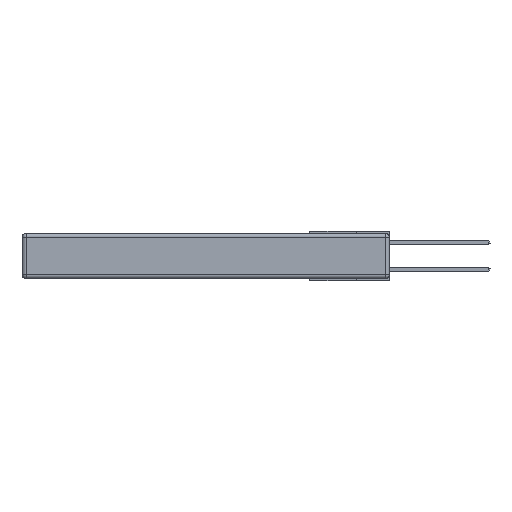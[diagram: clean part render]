
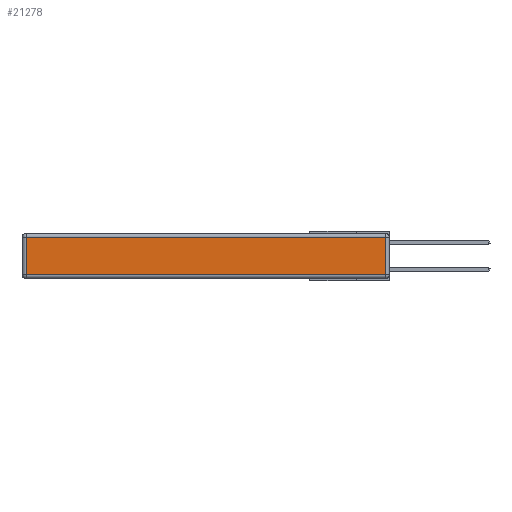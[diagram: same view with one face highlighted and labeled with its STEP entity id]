
A CAD part, left-side view. The second image highlights one B-rep face of the part: STEP entity #21278.
In plain terms, the highlighted planar face has unit normal (-1, 0, 0).
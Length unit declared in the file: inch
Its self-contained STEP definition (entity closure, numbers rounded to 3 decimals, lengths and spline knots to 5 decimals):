
#412 = ORIENTED_EDGE ( 'NONE', *, *, #29593, .T. ) ;
#1567 = VECTOR ( 'NONE', #12972, 39.37008 ) ;
#4146 = DIRECTION ( 'NONE',  ( -1., 0., 0. ) ) ;
#5106 = ORIENTED_EDGE ( 'NONE', *, *, #32100, .T. ) ;
#6417 = EDGE_LOOP ( 'NONE', ( #17326, #412, #8939, #5106 ) ) ;
#7132 = DIRECTION ( 'NONE',  ( 0., 0., -1. ) ) ;
#8939 = ORIENTED_EDGE ( 'NONE', *, *, #25237, .T. ) ;
#10039 = AXIS2_PLACEMENT_3D ( 'NONE', #23239, #4146, #11400 ) ;
#10421 = CARTESIAN_POINT ( 'NONE',  ( 0., 0.03, -0.343 ) ) ;
#10767 = CARTESIAN_POINT ( 'NONE',  ( 0., 2.75, -0.03 ) ) ;
#10838 = CARTESIAN_POINT ( 'NONE',  ( 0., 2.72, -0.313 ) ) ;
#11400 = DIRECTION ( 'NONE',  ( 0., 0., 1. ) ) ;
#12477 = CARTESIAN_POINT ( 'NONE',  ( 0., 0.03, -0.03 ) ) ;
#12972 = DIRECTION ( 'NONE',  ( 0., 0., 1. ) ) ;
#14260 = VERTEX_POINT ( 'NONE', #12477 ) ;
#15559 = VERTEX_POINT ( 'NONE', #24708 ) ;
#16966 = LINE ( 'NONE', #21399, #31125 ) ;
#17006 = CARTESIAN_POINT ( 'NONE',  ( 0., 0.03, -0.313 ) ) ;
#17326 = ORIENTED_EDGE ( 'NONE', *, *, #28165, .T. ) ;
#17914 = LINE ( 'NONE', #10767, #19088 ) ;
#19088 = VECTOR ( 'NONE', #28334, 39.37008 ) ;
#19495 = DIRECTION ( 'NONE',  ( 0., -1., 0. ) ) ;
#21278 = ADVANCED_FACE ( 'NONE', ( #31841 ), #28628, .T. ) ;
#21399 = CARTESIAN_POINT ( 'NONE',  ( 0., 0., -0.313 ) ) ;
#22134 = CARTESIAN_POINT ( 'NONE',  ( 0., 2.72, -0.343 ) ) ;
#23239 = CARTESIAN_POINT ( 'NONE',  ( 0., 0., -0.343 ) ) ;
#24520 = VERTEX_POINT ( 'NONE', #17006 ) ;
#24537 = LINE ( 'NONE', #22134, #31227 ) ;
#24708 = CARTESIAN_POINT ( 'NONE',  ( 0., 2.72, -0.03 ) ) ;
#25237 = EDGE_CURVE ( 'NONE', #14260, #15559, #17914, .T. ) ;
#28165 = EDGE_CURVE ( 'NONE', #32360, #24520, #16966, .T. ) ;
#28334 = DIRECTION ( 'NONE',  ( 0., 1., 0. ) ) ;
#28628 = PLANE ( 'NONE',  #10039 ) ;
#29593 = EDGE_CURVE ( 'NONE', #24520, #14260, #31034, .T. ) ;
#31034 = LINE ( 'NONE', #10421, #1567 ) ;
#31125 = VECTOR ( 'NONE', #19495, 39.37008 ) ;
#31227 = VECTOR ( 'NONE', #7132, 39.37008 ) ;
#31841 = FACE_OUTER_BOUND ( 'NONE', #6417, .T. ) ;
#32100 = EDGE_CURVE ( 'NONE', #15559, #32360, #24537, .T. ) ;
#32360 = VERTEX_POINT ( 'NONE', #10838 ) ;
